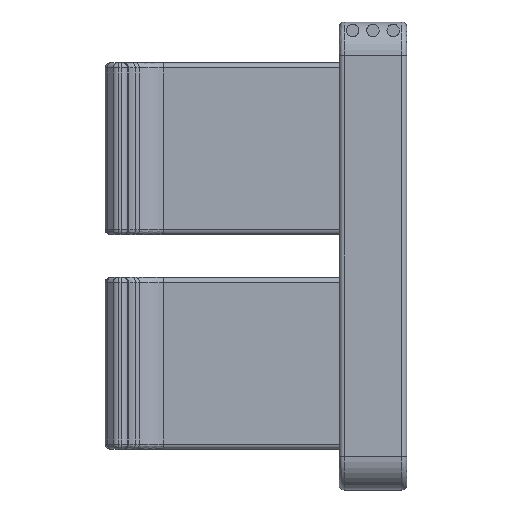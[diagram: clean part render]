
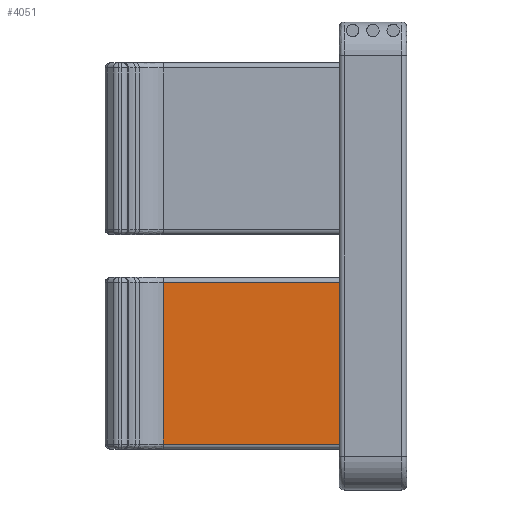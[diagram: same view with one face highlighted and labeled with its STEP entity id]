
A CAD part, left-side view. The second image highlights one B-rep face of the part: STEP entity #4051.
In plain terms, the highlighted planar face has unit normal (-1, 0, 0).
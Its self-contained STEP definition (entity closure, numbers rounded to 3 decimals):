
#59 = CARTESIAN_POINT ( 'NONE',  ( 34.098, 41.413, -34.631 ) ) ;
#365 = LINE ( 'NONE', #59, #1705 ) ;
#726 = VERTEX_POINT ( 'NONE', #5299 ) ;
#1314 = ORIENTED_EDGE ( 'NONE', *, *, #4205, .T. ) ;
#1334 = EDGE_LOOP ( 'NONE', ( #1314, #3926, #3754, #3116 ) ) ;
#1399 = CARTESIAN_POINT ( 'NONE',  ( 34.098, 7.884, -3.925 ) ) ;
#1466 = CARTESIAN_POINT ( 'NONE',  ( 34.098, 0., -34.631 ) ) ;
#1504 = PLANE ( 'NONE',  #1604 ) ;
#1604 = AXIS2_PLACEMENT_3D ( 'NONE', #1466, #5536, #2508 ) ;
#1705 = VECTOR ( 'NONE', #3068, 1000. ) ;
#2036 = LINE ( 'NONE', #2628, #4549 ) ;
#2172 = EDGE_CURVE ( 'NONE', #2886, #3520, #5859, .T. ) ;
#2508 = DIRECTION ( 'NONE',  ( 0., 0., 1. ) ) ;
#2573 = CARTESIAN_POINT ( 'NONE',  ( 34.098, 7.884, -27.825 ) ) ;
#2628 = CARTESIAN_POINT ( 'NONE',  ( 34.098, 0., -3.925 ) ) ;
#2886 = VERTEX_POINT ( 'NONE', #1399 ) ;
#2971 = VECTOR ( 'NONE', #6465, 1000. ) ;
#3068 = DIRECTION ( 'NONE',  ( 0., 0., -1. ) ) ;
#3116 = ORIENTED_EDGE ( 'NONE', *, *, #2172, .F. ) ;
#3338 = VERTEX_POINT ( 'NONE', #5166 ) ;
#3420 = CARTESIAN_POINT ( 'NONE',  ( 34.098, 7.884, -34.631 ) ) ;
#3519 = EDGE_CURVE ( 'NONE', #726, #3520, #3702, .T. ) ;
#3520 = VERTEX_POINT ( 'NONE', #2573 ) ;
#3536 = VECTOR ( 'NONE', #6123, 1000. ) ;
#3702 = LINE ( 'NONE', #5609, #3536 ) ;
#3754 = ORIENTED_EDGE ( 'NONE', *, *, #3519, .T. ) ;
#3926 = ORIENTED_EDGE ( 'NONE', *, *, #6252, .T. ) ;
#4051 = ADVANCED_FACE ( 'NONE', ( #5377 ), #1504, .F. ) ;
#4205 = EDGE_CURVE ( 'NONE', #2886, #3338, #2036, .T. ) ;
#4549 = VECTOR ( 'NONE', #5639, 1000. ) ;
#5166 = CARTESIAN_POINT ( 'NONE',  ( 34.098, 41.413, -3.925 ) ) ;
#5299 = CARTESIAN_POINT ( 'NONE',  ( 34.098, 41.413, -27.825 ) ) ;
#5377 = FACE_OUTER_BOUND ( 'NONE', #1334, .T. ) ;
#5536 = DIRECTION ( 'NONE',  ( 1., 0., 0. ) ) ;
#5609 = CARTESIAN_POINT ( 'NONE',  ( 34.098, 0., -27.825 ) ) ;
#5639 = DIRECTION ( 'NONE',  ( 0., 1., 0. ) ) ;
#5859 = LINE ( 'NONE', #3420, #2971 ) ;
#6123 = DIRECTION ( 'NONE',  ( 0., -1., 0. ) ) ;
#6252 = EDGE_CURVE ( 'NONE', #3338, #726, #365, .T. ) ;
#6465 = DIRECTION ( 'NONE',  ( 0., 0., -1. ) ) ;
